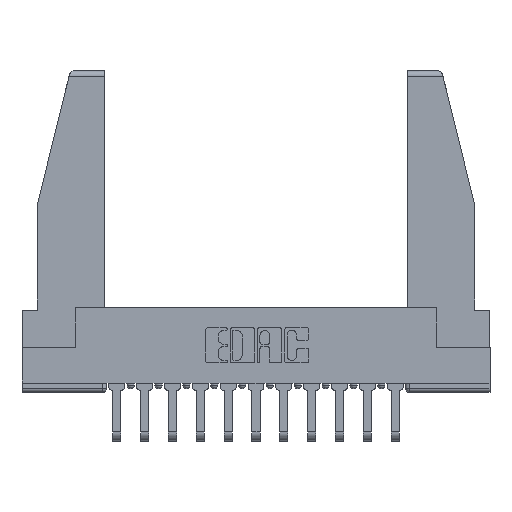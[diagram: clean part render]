
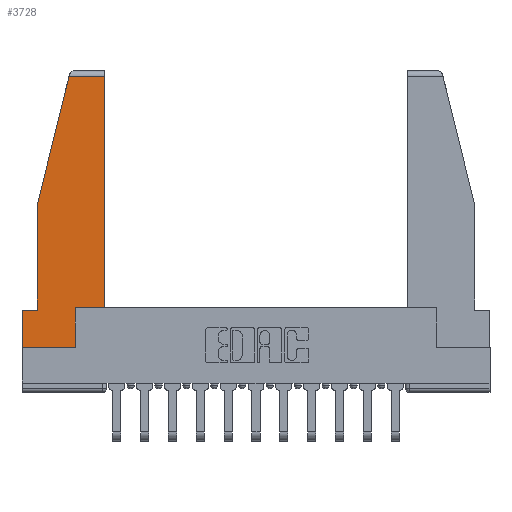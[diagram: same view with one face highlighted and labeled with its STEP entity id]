
A CAD part, top view. The second image highlights one B-rep face of the part: STEP entity #3728.
In plain terms, the highlighted planar face has unit normal (0, 0, 1).
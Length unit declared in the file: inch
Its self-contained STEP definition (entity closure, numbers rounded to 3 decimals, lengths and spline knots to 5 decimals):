
#187 = VERTEX_POINT ( 'NONE', #13245 ) ;
#283 = LINE ( 'NONE', #15641, #6561 ) ;
#481 = EDGE_LOOP ( 'NONE', ( #13143, #2299, #11192, #12227, #4325, #9716, #11068, #5054, #4277 ) ) ;
#582 = CARTESIAN_POINT ( 'NONE',  ( 0.297, 0., 0. ) ) ;
#599 = EDGE_CURVE ( 'NONE', #15527, #5165, #9496, .T. ) ;
#722 = VERTEX_POINT ( 'NONE', #8158 ) ;
#736 = EDGE_CURVE ( 'NONE', #5165, #722, #11962, .T. ) ;
#1056 = DIRECTION ( 'NONE',  ( 0., 1., 0. ) ) ;
#1495 = LINE ( 'NONE', #8671, #5120 ) ;
#2039 = LINE ( 'NONE', #8826, #14615 ) ;
#2277 = CARTESIAN_POINT ( 'NONE',  ( 0.297, 0.223, 0. ) ) ;
#2299 = ORIENTED_EDGE ( 'NONE', *, *, #11885, .T. ) ;
#3199 = VECTOR ( 'NONE', #6299, 39.37008 ) ;
#3323 = VERTEX_POINT ( 'NONE', #11996 ) ;
#3369 = EDGE_CURVE ( 'NONE', #11309, #10907, #9685, .T. ) ;
#3528 = AXIS2_PLACEMENT_3D ( 'NONE', #13572, #7492, #8967 ) ;
#3560 = VERTEX_POINT ( 'NONE', #7117 ) ;
#3728 = ADVANCED_FACE ( 'NONE', ( #12473 ), #12281, .T. ) ;
#4200 = EDGE_CURVE ( 'NONE', #10907, #3560, #14642, .T. ) ;
#4277 = ORIENTED_EDGE ( 'NONE', *, *, #4200, .T. ) ;
#4325 = ORIENTED_EDGE ( 'NONE', *, *, #736, .T. ) ;
#5054 = ORIENTED_EDGE ( 'NONE', *, *, #3369, .T. ) ;
#5092 = VERTEX_POINT ( 'NONE', #11693 ) ;
#5120 = VECTOR ( 'NONE', #7413, 39.37008 ) ;
#5165 = VERTEX_POINT ( 'NONE', #10378 ) ;
#5539 = CARTESIAN_POINT ( 'NONE',  ( 0.086, 0.8, 0. ) ) ;
#5670 = VECTOR ( 'NONE', #12827, 39.37008 ) ;
#6016 = VECTOR ( 'NONE', #12787, 39.37008 ) ;
#6027 = VECTOR ( 'NONE', #15444, 39.37008 ) ;
#6299 = DIRECTION ( 'NONE',  ( 1., 0., 0. ) ) ;
#6561 = VECTOR ( 'NONE', #8121, 39.37008 ) ;
#6679 = CARTESIAN_POINT ( 'NONE',  ( 0.086, 0.8, 0. ) ) ;
#6778 = LINE ( 'NONE', #11516, #6016 ) ;
#6927 = CARTESIAN_POINT ( 'NONE',  ( 0., 0.21, 0. ) ) ;
#7117 = CARTESIAN_POINT ( 'NONE',  ( 0.461, 0.223, 0. ) ) ;
#7413 = DIRECTION ( 'NONE',  ( 0., 1., 0. ) ) ;
#7492 = DIRECTION ( 'NONE',  ( 0., 0., 1. ) ) ;
#7778 = DIRECTION ( 'NONE',  ( -1., 0., 0. ) ) ;
#8121 = DIRECTION ( 'NONE',  ( -0.239, -0.971, 0. ) ) ;
#8158 = CARTESIAN_POINT ( 'NONE',  ( 0., 0.21, 0. ) ) ;
#8367 = CARTESIAN_POINT ( 'NONE',  ( 0.297, 0., 0. ) ) ;
#8671 = CARTESIAN_POINT ( 'NONE',  ( 0.461, 0.223, 0. ) ) ;
#8826 = CARTESIAN_POINT ( 'NONE',  ( 0., 1.52, 0. ) ) ;
#8967 = DIRECTION ( 'NONE',  ( 1., 0., 0. ) ) ;
#9328 = LINE ( 'NONE', #12031, #15234 ) ;
#9496 = LINE ( 'NONE', #5539, #5670 ) ;
#9685 = LINE ( 'NONE', #8367, #11765 ) ;
#9716 = ORIENTED_EDGE ( 'NONE', *, *, #12651, .T. ) ;
#10071 = EDGE_CURVE ( 'NONE', #3560, #5092, #1495, .T. ) ;
#10378 = CARTESIAN_POINT ( 'NONE',  ( 0.086, 0.21, 0. ) ) ;
#10516 = EDGE_CURVE ( 'NONE', #187, #11309, #9328, .T. ) ;
#10907 = VERTEX_POINT ( 'NONE', #2277 ) ;
#11068 = ORIENTED_EDGE ( 'NONE', *, *, #10516, .T. ) ;
#11192 = ORIENTED_EDGE ( 'NONE', *, *, #12778, .T. ) ;
#11309 = VERTEX_POINT ( 'NONE', #582 ) ;
#11516 = CARTESIAN_POINT ( 'NONE',  ( 0., 0.21, 0. ) ) ;
#11693 = CARTESIAN_POINT ( 'NONE',  ( 0.461, 1.52, 0. ) ) ;
#11765 = VECTOR ( 'NONE', #1056, 39.37008 ) ;
#11885 = EDGE_CURVE ( 'NONE', #5092, #3323, #2039, .T. ) ;
#11962 = LINE ( 'NONE', #6927, #6027 ) ;
#11996 = CARTESIAN_POINT ( 'NONE',  ( 0.2636, 1.52, 0. ) ) ;
#12031 = CARTESIAN_POINT ( 'NONE',  ( 0., 0., 0. ) ) ;
#12227 = ORIENTED_EDGE ( 'NONE', *, *, #599, .T. ) ;
#12281 = PLANE ( 'NONE',  #3528 ) ;
#12473 = FACE_OUTER_BOUND ( 'NONE', #481, .T. ) ;
#12651 = EDGE_CURVE ( 'NONE', #722, #187, #6778, .T. ) ;
#12778 = EDGE_CURVE ( 'NONE', #3323, #15527, #283, .T. ) ;
#12787 = DIRECTION ( 'NONE',  ( 0., -1., 0. ) ) ;
#12827 = DIRECTION ( 'NONE',  ( 0., -1., 0. ) ) ;
#13143 = ORIENTED_EDGE ( 'NONE', *, *, #10071, .T. ) ;
#13245 = CARTESIAN_POINT ( 'NONE',  ( 0., 0., 0. ) ) ;
#13359 = CARTESIAN_POINT ( 'NONE',  ( 0.297, 0.223, 0. ) ) ;
#13572 = CARTESIAN_POINT ( 'NONE',  ( 0., 0., 0. ) ) ;
#14388 = DIRECTION ( 'NONE',  ( 1., 0., 0. ) ) ;
#14615 = VECTOR ( 'NONE', #7778, 39.37008 ) ;
#14642 = LINE ( 'NONE', #13359, #3199 ) ;
#15234 = VECTOR ( 'NONE', #14388, 39.37008 ) ;
#15444 = DIRECTION ( 'NONE',  ( -1., 0., 0. ) ) ;
#15527 = VERTEX_POINT ( 'NONE', #6679 ) ;
#15641 = CARTESIAN_POINT ( 'NONE',  ( 0.271, 1.55, 0. ) ) ;
